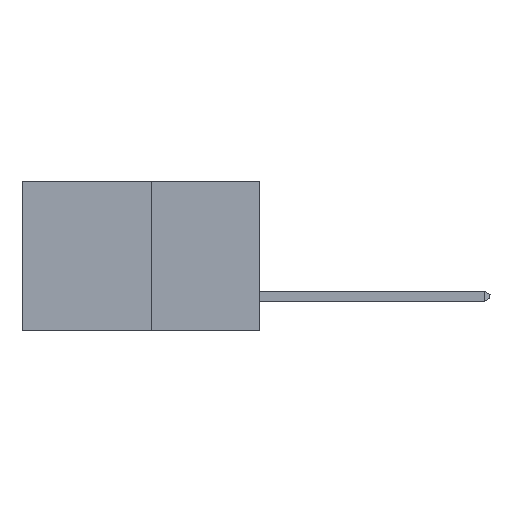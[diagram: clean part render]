
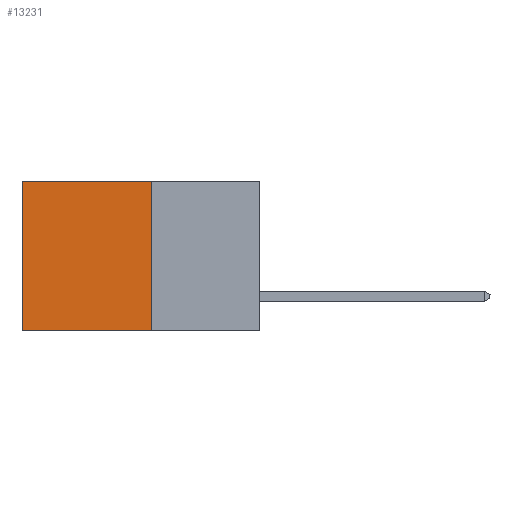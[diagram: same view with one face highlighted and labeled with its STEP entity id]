
A CAD part, left-side view. The second image highlights one B-rep face of the part: STEP entity #13231.
In plain terms, the highlighted planar face has unit normal (-1, 0, 0).
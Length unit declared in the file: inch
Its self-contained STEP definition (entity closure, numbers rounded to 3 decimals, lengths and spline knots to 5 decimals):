
#1358 = ORIENTED_EDGE ( 'NONE', *, *, #15922, .F. ) ;
#1498 = DIRECTION ( 'NONE',  ( 0., 0., -1. ) ) ;
#2078 = VERTEX_POINT ( 'NONE', #4899 ) ;
#2961 = EDGE_CURVE ( 'NONE', #2078, #3023, #16639, .T. ) ;
#2987 = EDGE_CURVE ( 'NONE', #3023, #15200, #13308, .T. ) ;
#3023 = VERTEX_POINT ( 'NONE', #11134 ) ;
#3118 = CARTESIAN_POINT ( 'NONE',  ( 0.277, 0.27, -0.37 ) ) ;
#3300 = VECTOR ( 'NONE', #5300, 39.37008 ) ;
#3663 = VECTOR ( 'NONE', #13034, 39.37008 ) ;
#4217 = VERTEX_POINT ( 'NONE', #5848 ) ;
#4899 = CARTESIAN_POINT ( 'NONE',  ( 0.277, 0.27, 0. ) ) ;
#5300 = DIRECTION ( 'NONE',  ( 0., 1., 0. ) ) ;
#5848 = CARTESIAN_POINT ( 'NONE',  ( 0.277, 0.27, -0.37 ) ) ;
#6906 = LINE ( 'NONE', #11812, #3300 ) ;
#7190 = PLANE ( 'NONE',  #9954 ) ;
#7324 = ORIENTED_EDGE ( 'NONE', *, *, #2987, .T. ) ;
#8020 = FACE_OUTER_BOUND ( 'NONE', #16968, .T. ) ;
#8526 = DIRECTION ( 'NONE',  ( 0., 0., -1. ) ) ;
#9545 = ORIENTED_EDGE ( 'NONE', *, *, #2961, .T. ) ;
#9954 = AXIS2_PLACEMENT_3D ( 'NONE', #3118, #16137, #8526 ) ;
#10621 = EDGE_CURVE ( 'NONE', #2078, #4217, #12767, .T. ) ;
#11134 = CARTESIAN_POINT ( 'NONE',  ( 0.277, 0.59, 0. ) ) ;
#11812 = CARTESIAN_POINT ( 'NONE',  ( 0.277, 0.27, -0.37 ) ) ;
#12381 = VECTOR ( 'NONE', #1498, 39.37008 ) ;
#12767 = LINE ( 'NONE', #15907, #12381 ) ;
#13034 = DIRECTION ( 'NONE',  ( 0., 0., -1. ) ) ;
#13090 = CARTESIAN_POINT ( 'NONE',  ( 0.277, 0.59, -0.37 ) ) ;
#13231 = ADVANCED_FACE ( 'NONE', ( #8020 ), #7190, .F. ) ;
#13308 = LINE ( 'NONE', #13090, #3663 ) ;
#13715 = VECTOR ( 'NONE', #13997, 39.37008 ) ;
#13997 = DIRECTION ( 'NONE',  ( 0., 1., 0. ) ) ;
#14039 = CARTESIAN_POINT ( 'NONE',  ( 0.277, 0.27, 0. ) ) ;
#14282 = CARTESIAN_POINT ( 'NONE',  ( 0.277, 0.59, -0.37 ) ) ;
#15200 = VERTEX_POINT ( 'NONE', #14282 ) ;
#15801 = ORIENTED_EDGE ( 'NONE', *, *, #10621, .F. ) ;
#15907 = CARTESIAN_POINT ( 'NONE',  ( 0.277, 0.27, -0.37 ) ) ;
#15922 = EDGE_CURVE ( 'NONE', #4217, #15200, #6906, .T. ) ;
#16137 = DIRECTION ( 'NONE',  ( 1., 0., 0. ) ) ;
#16639 = LINE ( 'NONE', #14039, #13715 ) ;
#16968 = EDGE_LOOP ( 'NONE', ( #7324, #1358, #15801, #9545 ) ) ;
